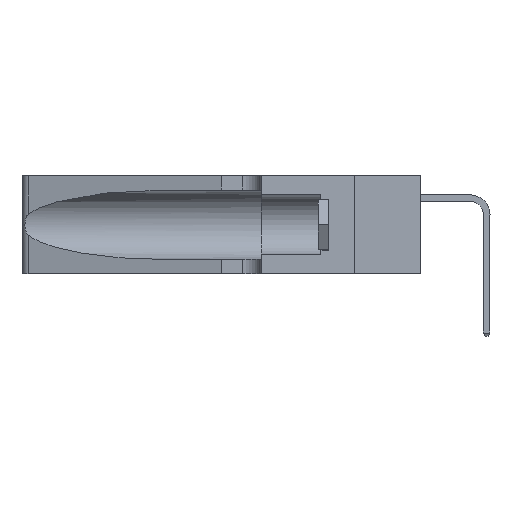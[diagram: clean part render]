
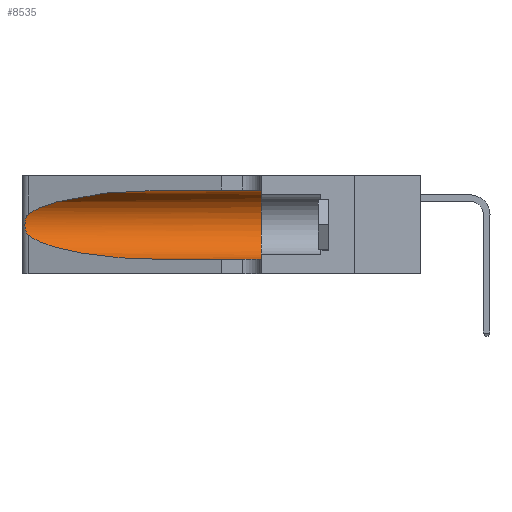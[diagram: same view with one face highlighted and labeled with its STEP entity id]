
A CAD part, left-side view. The second image highlights one B-rep face of the part: STEP entity #8535.
In plain terms, the highlighted cylindrical face has radius 3.308 mm (diameter 6.617 mm), a partial arc.
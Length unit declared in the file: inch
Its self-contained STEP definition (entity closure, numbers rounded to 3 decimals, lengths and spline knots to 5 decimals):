
#26 = LINE ( 'NONE', #17385, #15789 ) ;
#31 = CARTESIAN_POINT ( 'NONE',  ( 0.18966, 0.96281, 0.05475 ) ) ;
#208 = ORIENTED_EDGE ( 'NONE', *, *, #7854, .T. ) ;
#668 = CARTESIAN_POINT ( 'NONE',  ( 0.25555, 1.22994, 0.2215 ) ) ;
#687 = ORIENTED_EDGE ( 'NONE', *, *, #10913, .T. ) ;
#740 = CARTESIAN_POINT ( 'NONE',  ( 0.25487, 1.22718, 0.14631 ) ) ;
#903 = DIRECTION ( 'NONE',  ( 0., 1., 0. ) ) ;
#1432 = ORIENTED_EDGE ( 'NONE', *, *, #11285, .T. ) ;
#1453 = CARTESIAN_POINT ( 'NONE',  ( 0.1305, 0.35, 0.05475 ) ) ;
#1742 =( BOUNDED_CURVE ( )  B_SPLINE_CURVE ( 3, ( #7030, #16064, #8570, #19024 ),
 .UNSPECIFIED., .F., .F. ) 
 B_SPLINE_CURVE_WITH_KNOTS ( ( 4, 4 ),
 ( 1.5708, 2.84003 ),
 .UNSPECIFIED. ) 
 CURVE ( )  GEOMETRIC_REPRESENTATION_ITEM ( )  RATIONAL_B_SPLINE_CURVE ( ( 1., 0.87, 0.87, 1. ) ) 
 REPRESENTATION_ITEM ( '' )  );
#1850 = CARTESIAN_POINT ( 'NONE',  ( 0.25487, 1.22718, 0.14631 ) ) ;
#1884 = EDGE_CURVE ( 'NONE', #10409, #6209, #3142, .T. ) ;
#2222 = CARTESIAN_POINT ( 'NONE',  ( 0.25639, 1.23184, 0.21858 ) ) ;
#3142 = CIRCLE ( 'NONE', #8182, 0.13025 ) ;
#3789 = CARTESIAN_POINT ( 'NONE',  ( 0.25854, 1.2359, 0.20912 ) ) ;
#3828 = DIRECTION ( 'NONE',  ( 0., -1., 0. ) ) ;
#4266 = VERTEX_POINT ( 'NONE', #16926 ) ;
#4609 = CARTESIAN_POINT ( 'NONE',  ( 0.1305, 1.61858, 0.31525 ) ) ;
#4677 = CARTESIAN_POINT ( 'NONE',  ( 0.25487, 1.22718, 0.14631 ) ) ;
#5379 = CARTESIAN_POINT ( 'NONE',  ( 0.26075, 1.23896, 0.19203 ) ) ;
#5395 = CARTESIAN_POINT ( 'NONE',  ( 0.1305, 1.61858, 0.185 ) ) ;
#6209 = VERTEX_POINT ( 'NONE', #1453 ) ;
#6235 = VECTOR ( 'NONE', #7701, 39.37008 ) ;
#6826 = CYLINDRICAL_SURFACE ( 'NONE', #11436, 0.13025 ) ;
#6897 = CARTESIAN_POINT ( 'NONE',  ( 0.26017, 1.23833, 0.17102 ) ) ;
#7030 = CARTESIAN_POINT ( 'NONE',  ( 0.1305, 0.72297, 0.31525 ) ) ;
#7203 = DIRECTION ( 'NONE',  ( 0., 0., 1. ) ) ;
#7260 = EDGE_CURVE ( 'NONE', #18070, #4266, #1742, .T. ) ;
#7701 = DIRECTION ( 'NONE',  ( 0., -1., 0. ) ) ;
#7854 = EDGE_CURVE ( 'NONE', #12345, #6209, #26, .T. ) ;
#8182 = AXIS2_PLACEMENT_3D ( 'NONE', #13293, #903, #7203 ) ;
#8447 = CARTESIAN_POINT ( 'NONE',  ( 0.25789, 1.23486, 0.15765 ) ) ;
#8535 = ADVANCED_FACE ( 'NONE', ( #14853 ), #6826, .F. ) ;
#8570 = CARTESIAN_POINT ( 'NONE',  ( 0.2373, 1.15595, 0.28018 ) ) ;
#8678 = CARTESIAN_POINT ( 'NONE',  ( 0.1305, 0.35, 0.31525 ) ) ;
#9165 = EDGE_LOOP ( 'NONE', ( #11971, #687, #1432, #208, #18991, #12045 ) ) ;
#9985 = CARTESIAN_POINT ( 'NONE',  ( 0.25555, 1.22993, 0.14849 ) ) ;
#10409 = VERTEX_POINT ( 'NONE', #8678 ) ;
#10820 = CARTESIAN_POINT ( 'NONE',  ( 0.1305, 0.72297, 0.05475 ) ) ;
#10913 = EDGE_CURVE ( 'NONE', #4266, #19273, #17909, .T. ) ;
#10997 =( BOUNDED_CURVE ( )  B_SPLINE_CURVE ( 3, ( #4677, #19651, #31, #10820 ),
 .UNSPECIFIED., .F., .F. ) 
 B_SPLINE_CURVE_WITH_KNOTS ( ( 4, 4 ),
 ( 3.44316, 4.71239 ),
 .UNSPECIFIED. ) 
 CURVE ( )  GEOMETRIC_REPRESENTATION_ITEM ( )  RATIONAL_B_SPLINE_CURVE ( ( 1., 0.87, 0.87, 1. ) ) 
 REPRESENTATION_ITEM ( '' )  );
#11280 = EDGE_CURVE ( 'NONE', #18070, #10409, #14260, .T. ) ;
#11285 = EDGE_CURVE ( 'NONE', #19273, #12345, #10997, .T. ) ;
#11436 = AXIS2_PLACEMENT_3D ( 'NONE', #5395, #15875, #15951 ) ;
#11971 = ORIENTED_EDGE ( 'NONE', *, *, #7260, .T. ) ;
#12045 = ORIENTED_EDGE ( 'NONE', *, *, #11280, .F. ) ;
#12345 = VERTEX_POINT ( 'NONE', #17979 ) ;
#12916 = CARTESIAN_POINT ( 'NONE',  ( 0.25787, 1.23484, 0.2124 ) ) ;
#13293 = CARTESIAN_POINT ( 'NONE',  ( 0.1305, 0.35, 0.185 ) ) ;
#14260 = LINE ( 'NONE', #4609, #6235 ) ;
#14423 = CARTESIAN_POINT ( 'NONE',  ( 0.26018, 1.23835, 0.19895 ) ) ;
#14853 = FACE_OUTER_BOUND ( 'NONE', #9165, .T. ) ;
#15789 = VECTOR ( 'NONE', #3828, 39.37008 ) ;
#15875 = DIRECTION ( 'NONE',  ( 0., -1., 0. ) ) ;
#15938 = CARTESIAN_POINT ( 'NONE',  ( 0.26075, 1.23896, 0.178 ) ) ;
#15951 = DIRECTION ( 'NONE',  ( 0., 0., -1. ) ) ;
#16064 = CARTESIAN_POINT ( 'NONE',  ( 0.18966, 0.96281, 0.31525 ) ) ;
#16926 = CARTESIAN_POINT ( 'NONE',  ( 0.25487, 1.22718, 0.22369 ) ) ;
#17385 = CARTESIAN_POINT ( 'NONE',  ( 0.1305, 1.61858, 0.05475 ) ) ;
#17416 = CARTESIAN_POINT ( 'NONE',  ( 0.25856, 1.23593, 0.16098 ) ) ;
#17909 = B_SPLINE_CURVE_WITH_KNOTS ( 'NONE', 3,
 ( #18841, #668, #2222, #12916, #3789, #14423, #5379, #15938, #6897, #17416, #8447, #18903, #9985, #740 ),
 .UNSPECIFIED., .F., .F.,
 ( 4, 2, 2, 2, 2, 2, 4 ),
 ( 0., 0.00027, 0.00053, 0.00107, 0.0016, 0.00187, 0.00214 ),
 .UNSPECIFIED. ) ;
#17979 = CARTESIAN_POINT ( 'NONE',  ( 0.1305, 0.72297, 0.05475 ) ) ;
#18070 = VERTEX_POINT ( 'NONE', #18714 ) ;
#18714 = CARTESIAN_POINT ( 'NONE',  ( 0.1305, 0.72297, 0.31525 ) ) ;
#18841 = CARTESIAN_POINT ( 'NONE',  ( 0.25487, 1.22718, 0.22369 ) ) ;
#18903 = CARTESIAN_POINT ( 'NONE',  ( 0.25639, 1.23186, 0.15144 ) ) ;
#18991 = ORIENTED_EDGE ( 'NONE', *, *, #1884, .F. ) ;
#19024 = CARTESIAN_POINT ( 'NONE',  ( 0.25487, 1.22718, 0.22369 ) ) ;
#19273 = VERTEX_POINT ( 'NONE', #1850 ) ;
#19651 = CARTESIAN_POINT ( 'NONE',  ( 0.2373, 1.15595, 0.08982 ) ) ;
